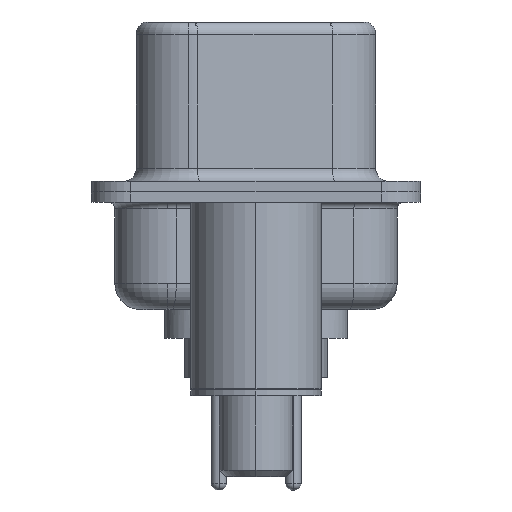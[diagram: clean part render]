
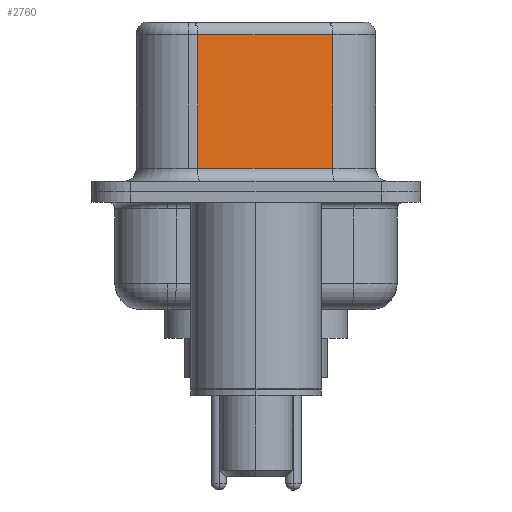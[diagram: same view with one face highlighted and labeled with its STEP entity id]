
A CAD part, left-side view. The second image highlights one B-rep face of the part: STEP entity #2760.
In plain terms, the highlighted planar face has unit normal (-0.985, -0.174, 0).
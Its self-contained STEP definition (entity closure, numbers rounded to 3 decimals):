
#391 = ORIENTED_EDGE ( 'NONE', *, *, #10085, .F. ) ;
#1163 = CARTESIAN_POINT ( 'NONE',  ( 4.58, -2.927, 0.9 ) ) ;
#1218 = DIRECTION ( 'NONE',  ( 0.174, -0.985, 0. ) ) ;
#2760 = ADVANCED_FACE ( 'NONE', ( #21116 ), #5294, .F. ) ;
#3518 = LINE ( 'NONE', #26170, #8446 ) ;
#4894 = DIRECTION ( 'NONE',  ( 0., 0., -1. ) ) ;
#5013 = VECTOR ( 'NONE', #4894, 1000. ) ;
#5294 = PLANE ( 'NONE',  #10543 ) ;
#5314 = VERTEX_POINT ( 'NONE', #20605 ) ;
#5555 = ORIENTED_EDGE ( 'NONE', *, *, #8325, .T. ) ;
#5885 = ORIENTED_EDGE ( 'NONE', *, *, #19190, .T. ) ;
#6225 = CARTESIAN_POINT ( 'NONE',  ( 4.58, -2.927, 6.52 ) ) ;
#6474 = EDGE_LOOP ( 'NONE', ( #391, #5555, #22422, #5885 ) ) ;
#6865 = VECTOR ( 'NONE', #10127, 1000. ) ;
#7471 = CARTESIAN_POINT ( 'NONE',  ( 4.58, -2.927, 6.02 ) ) ;
#8325 = EDGE_CURVE ( 'NONE', #25820, #10148, #22820, .T. ) ;
#8446 = VECTOR ( 'NONE', #1218, 1000. ) ;
#8978 = VERTEX_POINT ( 'NONE', #1163 ) ;
#9518 = CARTESIAN_POINT ( 'NONE',  ( 4.58, -2.927, 6.02 ) ) ;
#10085 = EDGE_CURVE ( 'NONE', #25820, #8978, #23322, .T. ) ;
#10127 = DIRECTION ( 'NONE',  ( 0., 0., -1. ) ) ;
#10148 = VERTEX_POINT ( 'NONE', #18450 ) ;
#10543 = AXIS2_PLACEMENT_3D ( 'NONE', #6225, #17203, #18797 ) ;
#10569 = LINE ( 'NONE', #11077, #5013 ) ;
#11077 = CARTESIAN_POINT ( 'NONE',  ( 3.67, 2.233, 6.52 ) ) ;
#11861 = VECTOR ( 'NONE', #21879, 1000. ) ;
#17203 = DIRECTION ( 'NONE',  ( 0.985, 0.174, 0. ) ) ;
#18450 = CARTESIAN_POINT ( 'NONE',  ( 3.67, 2.233, 6.02 ) ) ;
#18797 = DIRECTION ( 'NONE',  ( -0.174, 0.985, 0. ) ) ;
#19190 = EDGE_CURVE ( 'NONE', #5314, #8978, #3518, .T. ) ;
#20605 = CARTESIAN_POINT ( 'NONE',  ( 3.67, 2.233, 0.9 ) ) ;
#21116 = FACE_OUTER_BOUND ( 'NONE', #6474, .T. ) ;
#21879 = DIRECTION ( 'NONE',  ( -0.174, 0.985, 0. ) ) ;
#22422 = ORIENTED_EDGE ( 'NONE', *, *, #23132, .T. ) ;
#22820 = LINE ( 'NONE', #7471, #11861 ) ;
#23132 = EDGE_CURVE ( 'NONE', #10148, #5314, #10569, .T. ) ;
#23322 = LINE ( 'NONE', #26631, #6865 ) ;
#25820 = VERTEX_POINT ( 'NONE', #9518 ) ;
#26170 = CARTESIAN_POINT ( 'NONE',  ( 4.58, -2.927, 0.9 ) ) ;
#26631 = CARTESIAN_POINT ( 'NONE',  ( 4.58, -2.927, 6.52 ) ) ;
